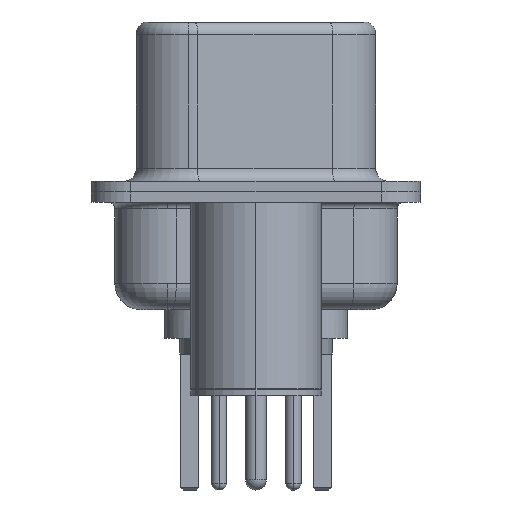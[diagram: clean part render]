
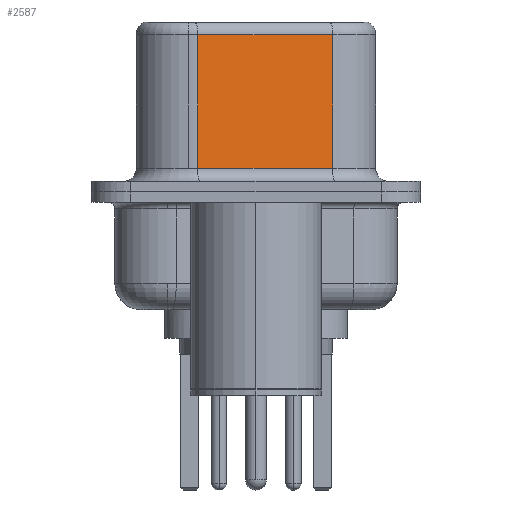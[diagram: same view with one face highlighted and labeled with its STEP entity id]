
A CAD part, left-side view. The second image highlights one B-rep face of the part: STEP entity #2587.
In plain terms, the highlighted planar face has unit normal (-0.985, -0.174, 0).
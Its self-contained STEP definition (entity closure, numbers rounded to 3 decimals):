
#992 = VECTOR ( 'NONE', #15420, 1000. ) ;
#1700 = ORIENTED_EDGE ( 'NONE', *, *, #15130, .T. ) ;
#1763 = DIRECTION ( 'NONE',  ( 0.985, 0.174, 0. ) ) ;
#2056 = VECTOR ( 'NONE', #8755, 1000. ) ;
#2587 = ADVANCED_FACE ( 'NONE', ( #10890 ), #11580, .F. ) ;
#2603 = LINE ( 'NONE', #20818, #18146 ) ;
#4193 = EDGE_CURVE ( 'NONE', #21586, #17296, #2603, .T. ) ;
#5380 = EDGE_CURVE ( 'NONE', #13527, #21586, #13017, .T. ) ;
#6556 = DIRECTION ( 'NONE',  ( 0.174, -0.985, 0. ) ) ;
#8755 = DIRECTION ( 'NONE',  ( 0., 0., -1. ) ) ;
#9723 = DIRECTION ( 'NONE',  ( -0.174, 0.985, 0. ) ) ;
#10168 = LINE ( 'NONE', #10242, #992 ) ;
#10242 = CARTESIAN_POINT ( 'NONE',  ( 4.585, -2.927, 6.02 ) ) ;
#10890 = FACE_OUTER_BOUND ( 'NONE', #25534, .T. ) ;
#11580 = PLANE ( 'NONE',  #14442 ) ;
#11815 = CARTESIAN_POINT ( 'NONE',  ( 3.675, 2.233, 0.9 ) ) ;
#13017 = LINE ( 'NONE', #14160, #25412 ) ;
#13093 = ORIENTED_EDGE ( 'NONE', *, *, #4193, .T. ) ;
#13116 = EDGE_CURVE ( 'NONE', #18008, #17296, #13451, .T. ) ;
#13451 = LINE ( 'NONE', #23128, #2056 ) ;
#13503 = ORIENTED_EDGE ( 'NONE', *, *, #5380, .T. ) ;
#13527 = VERTEX_POINT ( 'NONE', #16808 ) ;
#13623 = CARTESIAN_POINT ( 'NONE',  ( 4.585, -2.927, 6.52 ) ) ;
#14160 = CARTESIAN_POINT ( 'NONE',  ( 3.675, 2.233, 6.52 ) ) ;
#14442 = AXIS2_PLACEMENT_3D ( 'NONE', #13623, #1763, #9723 ) ;
#15130 = EDGE_CURVE ( 'NONE', #18008, #13527, #10168, .T. ) ;
#15420 = DIRECTION ( 'NONE',  ( -0.174, 0.985, 0. ) ) ;
#16808 = CARTESIAN_POINT ( 'NONE',  ( 3.675, 2.233, 6.02 ) ) ;
#17296 = VERTEX_POINT ( 'NONE', #26060 ) ;
#18008 = VERTEX_POINT ( 'NONE', #25709 ) ;
#18146 = VECTOR ( 'NONE', #6556, 1000. ) ;
#18619 = DIRECTION ( 'NONE',  ( 0., 0., -1. ) ) ;
#20494 = ORIENTED_EDGE ( 'NONE', *, *, #13116, .F. ) ;
#20818 = CARTESIAN_POINT ( 'NONE',  ( 4.585, -2.927, 0.9 ) ) ;
#21586 = VERTEX_POINT ( 'NONE', #11815 ) ;
#23128 = CARTESIAN_POINT ( 'NONE',  ( 4.585, -2.927, 6.52 ) ) ;
#25412 = VECTOR ( 'NONE', #18619, 1000. ) ;
#25534 = EDGE_LOOP ( 'NONE', ( #20494, #1700, #13503, #13093 ) ) ;
#25709 = CARTESIAN_POINT ( 'NONE',  ( 4.585, -2.927, 6.02 ) ) ;
#26060 = CARTESIAN_POINT ( 'NONE',  ( 4.585, -2.927, 0.9 ) ) ;
